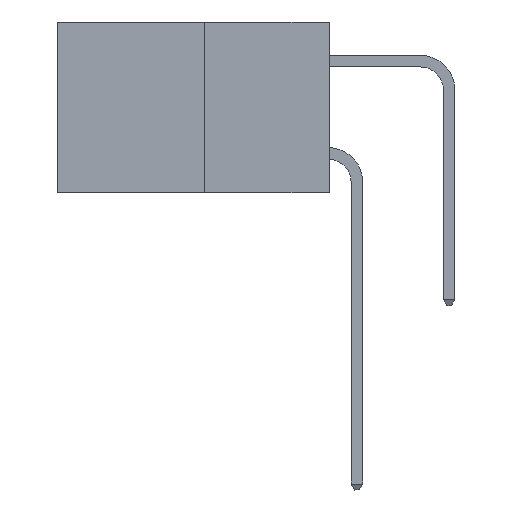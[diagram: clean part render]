
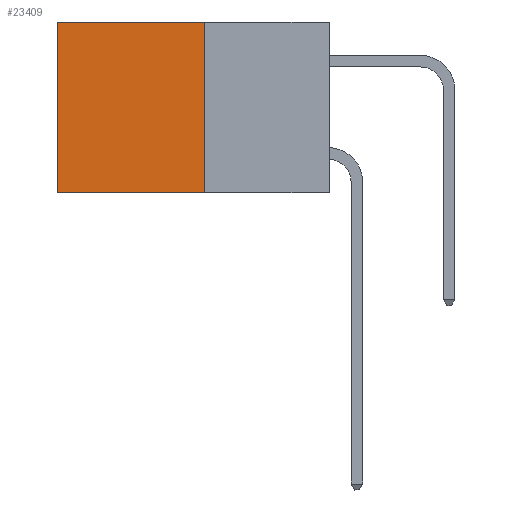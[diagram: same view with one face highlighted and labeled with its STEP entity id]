
A CAD part, left-side view. The second image highlights one B-rep face of the part: STEP entity #23409.
In plain terms, the highlighted planar face has unit normal (-1, 0, 0).
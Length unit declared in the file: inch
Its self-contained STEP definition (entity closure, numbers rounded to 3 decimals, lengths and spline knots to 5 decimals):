
#605 = VERTEX_POINT ( 'NONE', #9798 ) ;
#1330 = CARTESIAN_POINT ( 'NONE',  ( 0.277, 0.27, 0. ) ) ;
#2451 = EDGE_LOOP ( 'NONE', ( #14698, #3598, #26225, #27317 ) ) ;
#3370 = CARTESIAN_POINT ( 'NONE',  ( 0.277, 0.27, -0.37 ) ) ;
#3517 = EDGE_CURVE ( 'NONE', #26427, #18764, #22743, .T. ) ;
#3598 = ORIENTED_EDGE ( 'NONE', *, *, #10733, .F. ) ;
#4516 = CARTESIAN_POINT ( 'NONE',  ( 0.277, 0.59, -0.37 ) ) ;
#4743 = PLANE ( 'NONE',  #9140 ) ;
#5008 = LINE ( 'NONE', #3370, #26799 ) ;
#6397 = LINE ( 'NONE', #13171, #17660 ) ;
#9140 = AXIS2_PLACEMENT_3D ( 'NONE', #19539, #25871, #13279 ) ;
#9519 = VECTOR ( 'NONE', #22019, 39.37008 ) ;
#9798 = CARTESIAN_POINT ( 'NONE',  ( 0.277, 0.27, -0.37 ) ) ;
#10733 = EDGE_CURVE ( 'NONE', #605, #18764, #17114, .T. ) ;
#12141 = VECTOR ( 'NONE', #16041, 39.37008 ) ;
#13007 = EDGE_CURVE ( 'NONE', #15955, #26427, #6397, .T. ) ;
#13171 = CARTESIAN_POINT ( 'NONE',  ( 0.277, 0.27, 0. ) ) ;
#13279 = DIRECTION ( 'NONE',  ( 0., 0., -1. ) ) ;
#13921 = CARTESIAN_POINT ( 'NONE',  ( 0.277, 0.27, -0.37 ) ) ;
#14650 = EDGE_CURVE ( 'NONE', #15955, #605, #5008, .T. ) ;
#14698 = ORIENTED_EDGE ( 'NONE', *, *, #3517, .T. ) ;
#15542 = CARTESIAN_POINT ( 'NONE',  ( 0.277, 0.59, 0. ) ) ;
#15955 = VERTEX_POINT ( 'NONE', #1330 ) ;
#16041 = DIRECTION ( 'NONE',  ( 0., 1., 0. ) ) ;
#17114 = LINE ( 'NONE', #13921, #12141 ) ;
#17660 = VECTOR ( 'NONE', #25757, 39.37008 ) ;
#18764 = VERTEX_POINT ( 'NONE', #4516 ) ;
#19539 = CARTESIAN_POINT ( 'NONE',  ( 0.277, 0.27, -0.37 ) ) ;
#20194 = FACE_OUTER_BOUND ( 'NONE', #2451, .T. ) ;
#21800 = CARTESIAN_POINT ( 'NONE',  ( 0.277, 0.59, -0.37 ) ) ;
#22019 = DIRECTION ( 'NONE',  ( 0., 0., -1. ) ) ;
#22743 = LINE ( 'NONE', #21800, #9519 ) ;
#23409 = ADVANCED_FACE ( 'NONE', ( #20194 ), #4743, .F. ) ;
#24465 = DIRECTION ( 'NONE',  ( 0., 0., -1. ) ) ;
#25757 = DIRECTION ( 'NONE',  ( 0., 1., 0. ) ) ;
#25871 = DIRECTION ( 'NONE',  ( 1., 0., 0. ) ) ;
#26225 = ORIENTED_EDGE ( 'NONE', *, *, #14650, .F. ) ;
#26427 = VERTEX_POINT ( 'NONE', #15542 ) ;
#26799 = VECTOR ( 'NONE', #24465, 39.37008 ) ;
#27317 = ORIENTED_EDGE ( 'NONE', *, *, #13007, .T. ) ;
